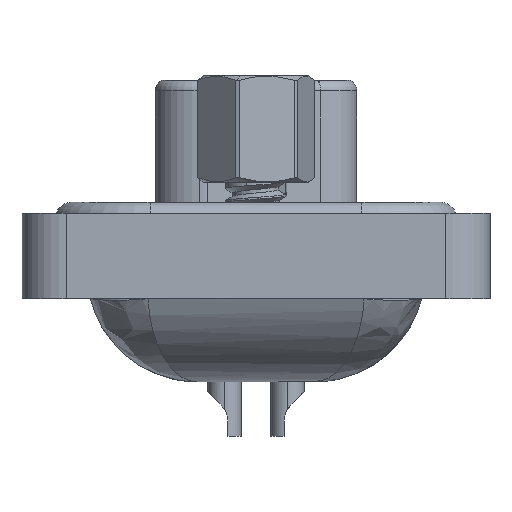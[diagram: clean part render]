
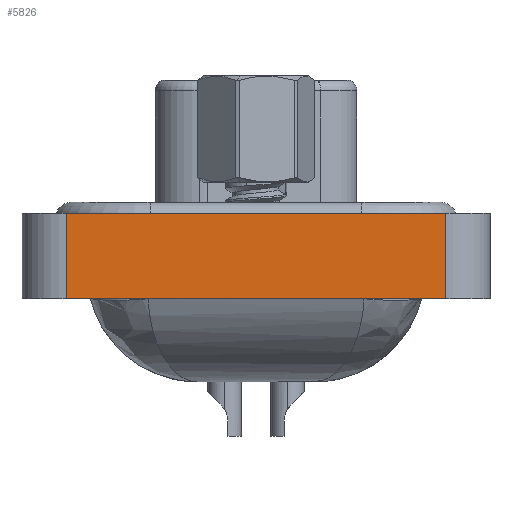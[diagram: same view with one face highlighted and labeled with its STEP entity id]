
A CAD part, left-side view. The second image highlights one B-rep face of the part: STEP entity #5826.
In plain terms, the highlighted planar face has unit normal (-1, 0, 0).
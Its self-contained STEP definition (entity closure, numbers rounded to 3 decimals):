
#433 = VERTEX_POINT ( 'NONE', #21842 ) ;
#2011 = CARTESIAN_POINT ( 'NONE',  ( -7.225, 8.55, 0.5 ) ) ;
#2934 = CARTESIAN_POINT ( 'NONE',  ( -7.225, -8.55, -3.35 ) ) ;
#2957 = DIRECTION ( 'NONE',  ( -1., 0., 0. ) ) ;
#3326 = CARTESIAN_POINT ( 'NONE',  ( -7.225, 8.55, -3.35 ) ) ;
#5549 = AXIS2_PLACEMENT_3D ( 'NONE', #22209, #2957, #11438 ) ;
#5826 = ADVANCED_FACE ( 'NONE', ( #26754 ), #15685, .T. ) ;
#6702 = EDGE_CURVE ( 'NONE', #24657, #22010, #12836, .T. ) ;
#7667 = CARTESIAN_POINT ( 'NONE',  ( -7.225, -8.55, 0.5 ) ) ;
#8225 = LINE ( 'NONE', #25262, #10777 ) ;
#8353 = VERTEX_POINT ( 'NONE', #12056 ) ;
#9552 = LINE ( 'NONE', #3326, #14001 ) ;
#9588 = DIRECTION ( 'NONE',  ( 0., 0., 1. ) ) ;
#9603 = VECTOR ( 'NONE', #16821, 1000. ) ;
#10777 = VECTOR ( 'NONE', #21272, 1000. ) ;
#11339 = EDGE_CURVE ( 'NONE', #8353, #433, #8225, .T. ) ;
#11438 = DIRECTION ( 'NONE',  ( 0., 0., 1. ) ) ;
#12056 = CARTESIAN_POINT ( 'NONE',  ( -7.225, 8.55, -3.35 ) ) ;
#12600 = EDGE_CURVE ( 'NONE', #8353, #24657, #9552, .T. ) ;
#12836 = LINE ( 'NONE', #16961, #9603 ) ;
#14001 = VECTOR ( 'NONE', #26702, 1000. ) ;
#14699 = VECTOR ( 'NONE', #9588, 1000. ) ;
#15685 = PLANE ( 'NONE',  #5549 ) ;
#15886 = ORIENTED_EDGE ( 'NONE', *, *, #19577, .T. ) ;
#16023 = ORIENTED_EDGE ( 'NONE', *, *, #12600, .F. ) ;
#16339 = ORIENTED_EDGE ( 'NONE', *, *, #6702, .F. ) ;
#16659 = ORIENTED_EDGE ( 'NONE', *, *, #11339, .T. ) ;
#16821 = DIRECTION ( 'NONE',  ( 0., -1., 0. ) ) ;
#16961 = CARTESIAN_POINT ( 'NONE',  ( -7.225, -8.55, 0.5 ) ) ;
#19577 = EDGE_CURVE ( 'NONE', #433, #22010, #22343, .T. ) ;
#21272 = DIRECTION ( 'NONE',  ( 0., -1., 0. ) ) ;
#21842 = CARTESIAN_POINT ( 'NONE',  ( -7.225, -8.55, -3.35 ) ) ;
#22010 = VERTEX_POINT ( 'NONE', #7667 ) ;
#22209 = CARTESIAN_POINT ( 'NONE',  ( -7.225, -8.55, -3.35 ) ) ;
#22343 = LINE ( 'NONE', #2934, #14699 ) ;
#24657 = VERTEX_POINT ( 'NONE', #2011 ) ;
#25262 = CARTESIAN_POINT ( 'NONE',  ( -7.225, -8.55, -3.35 ) ) ;
#26702 = DIRECTION ( 'NONE',  ( 0., 0., 1. ) ) ;
#26754 = FACE_OUTER_BOUND ( 'NONE', #27138, .T. ) ;
#27138 = EDGE_LOOP ( 'NONE', ( #15886, #16339, #16023, #16659 ) ) ;
